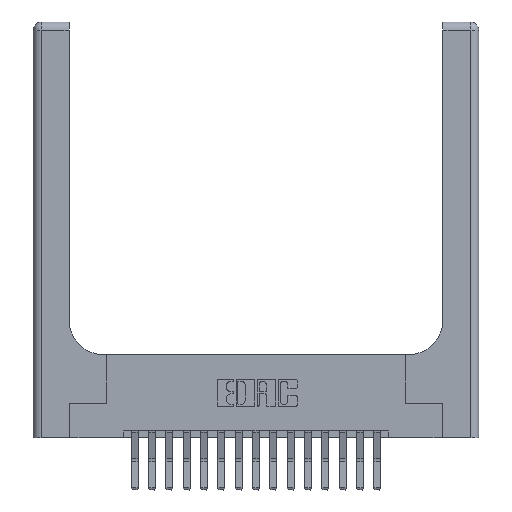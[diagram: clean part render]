
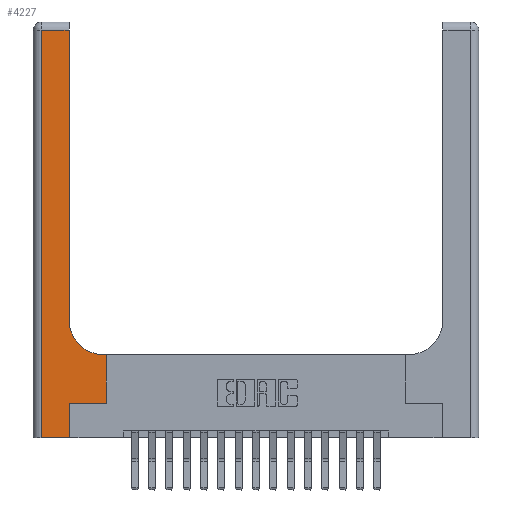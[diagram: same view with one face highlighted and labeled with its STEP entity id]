
A CAD part, top view. The second image highlights one B-rep face of the part: STEP entity #4227.
In plain terms, the highlighted planar face has unit normal (0, 0, 1).
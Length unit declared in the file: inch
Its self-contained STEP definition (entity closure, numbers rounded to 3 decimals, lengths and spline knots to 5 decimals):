
#165 = VERTEX_POINT ( 'NONE', #13885 ) ;
#406 = LINE ( 'NONE', #6337, #1240 ) ;
#1240 = VECTOR ( 'NONE', #18122, 39.37008 ) ;
#1593 = AXIS2_PLACEMENT_3D ( 'NONE', #10858, #15667, #2208 ) ;
#1728 = CARTESIAN_POINT ( 'NONE',  ( 0.265, 0., 0.37 ) ) ;
#1747 = ORIENTED_EDGE ( 'NONE', *, *, #4303, .T. ) ;
#1875 = DIRECTION ( 'NONE',  ( 0., -1., 0. ) ) ;
#2120 = VECTOR ( 'NONE', #1875, 39.37008 ) ;
#2208 = DIRECTION ( 'NONE',  ( 1., 0., 0. ) ) ;
#2814 = ORIENTED_EDGE ( 'NONE', *, *, #10517, .T. ) ;
#3023 = EDGE_CURVE ( 'NONE', #6909, #7137, #11379, .T. ) ;
#3226 = VERTEX_POINT ( 'NONE', #14758 ) ;
#3451 = CARTESIAN_POINT ( 'NONE',  ( 0.528, 0.25, 0.37 ) ) ;
#3509 = DIRECTION ( 'NONE',  ( 1., 0., 0. ) ) ;
#3814 = CARTESIAN_POINT ( 'NONE',  ( 0.26, 0.85, 0.37 ) ) ;
#3913 = DIRECTION ( 'NONE',  ( -1., 0., 0. ) ) ;
#4227 = ADVANCED_FACE ( 'NONE', ( #18217 ), #15396, .F. ) ;
#4303 = EDGE_CURVE ( 'NONE', #10622, #6909, #406, .T. ) ;
#4566 = CARTESIAN_POINT ( 'NONE',  ( 0.06, 2.94, 0.37 ) ) ;
#4660 = ORIENTED_EDGE ( 'NONE', *, *, #9718, .T. ) ;
#5021 = CARTESIAN_POINT ( 'NONE',  ( 0.265, 0.25, 0.37 ) ) ;
#5170 = EDGE_CURVE ( 'NONE', #15595, #15411, #8668, .T. ) ;
#5371 = DIRECTION ( 'NONE',  ( -1., 0., 0. ) ) ;
#5486 = CARTESIAN_POINT ( 'NONE',  ( 0., 2.94, 0.37 ) ) ;
#5850 = EDGE_LOOP ( 'NONE', ( #1747, #8269, #16518, #4660, #14651, #16987, #2814, #18423, #16940 ) ) ;
#6337 = CARTESIAN_POINT ( 'NONE',  ( 0.26, 3., 0.37 ) ) ;
#6622 = CARTESIAN_POINT ( 'NONE',  ( 0.26, 2.94, 0.37 ) ) ;
#6909 = VERTEX_POINT ( 'NONE', #6622 ) ;
#7126 = CARTESIAN_POINT ( 'NONE',  ( 0.26, 0.6, 0.37 ) ) ;
#7137 = VERTEX_POINT ( 'NONE', #4566 ) ;
#7566 = VERTEX_POINT ( 'NONE', #3451 ) ;
#7659 = DIRECTION ( 'NONE',  ( 0., 1., 0. ) ) ;
#7950 = LINE ( 'NONE', #1728, #9952 ) ;
#8118 = CIRCLE ( 'NONE', #1593, 0.25 ) ;
#8269 = ORIENTED_EDGE ( 'NONE', *, *, #3023, .T. ) ;
#8276 = VECTOR ( 'NONE', #11025, 39.37008 ) ;
#8297 = DIRECTION ( 'NONE',  ( 0., 1., 0. ) ) ;
#8310 = CARTESIAN_POINT ( 'NONE',  ( 0.51, 0.6, 0.37 ) ) ;
#8386 = EDGE_CURVE ( 'NONE', #15411, #10622, #8118, .T. ) ;
#8668 = LINE ( 'NONE', #7126, #15766 ) ;
#8744 = EDGE_CURVE ( 'NONE', #165, #11855, #7950, .T. ) ;
#9235 = DIRECTION ( 'NONE',  ( -1., 0., 0. ) ) ;
#9718 = EDGE_CURVE ( 'NONE', #3226, #165, #18427, .T. ) ;
#9952 = VECTOR ( 'NONE', #7659, 39.37008 ) ;
#10517 = EDGE_CURVE ( 'NONE', #7566, #15595, #17178, .T. ) ;
#10622 = VERTEX_POINT ( 'NONE', #3814 ) ;
#10858 = CARTESIAN_POINT ( 'NONE',  ( 0.51, 0.85, 0.37 ) ) ;
#11025 = DIRECTION ( 'NONE',  ( 1., 0., 0. ) ) ;
#11379 = LINE ( 'NONE', #5486, #18909 ) ;
#11855 = VERTEX_POINT ( 'NONE', #12189 ) ;
#12189 = CARTESIAN_POINT ( 'NONE',  ( 0.265, 0.25, 0.37 ) ) ;
#12594 = CARTESIAN_POINT ( 'NONE',  ( 0., 0., 0.37 ) ) ;
#13567 = CARTESIAN_POINT ( 'NONE',  ( 0., 3., 0.37 ) ) ;
#13885 = CARTESIAN_POINT ( 'NONE',  ( 0.265, 0., 0.37 ) ) ;
#13955 = LINE ( 'NONE', #16965, #2120 ) ;
#14616 = VECTOR ( 'NONE', #3509, 39.37008 ) ;
#14651 = ORIENTED_EDGE ( 'NONE', *, *, #8744, .T. ) ;
#14758 = CARTESIAN_POINT ( 'NONE',  ( 0.06, 0., 0.37 ) ) ;
#15134 = AXIS2_PLACEMENT_3D ( 'NONE', #13567, #16574, #9235 ) ;
#15396 = PLANE ( 'NONE',  #15134 ) ;
#15411 = VERTEX_POINT ( 'NONE', #8310 ) ;
#15595 = VERTEX_POINT ( 'NONE', #15928 ) ;
#15667 = DIRECTION ( 'NONE',  ( 0., 0., -1. ) ) ;
#15766 = VECTOR ( 'NONE', #5371, 39.37008 ) ;
#15928 = CARTESIAN_POINT ( 'NONE',  ( 0.528, 0.6, 0.37 ) ) ;
#16498 = VECTOR ( 'NONE', #8297, 39.37008 ) ;
#16518 = ORIENTED_EDGE ( 'NONE', *, *, #18689, .T. ) ;
#16540 = EDGE_CURVE ( 'NONE', #11855, #7566, #18278, .T. ) ;
#16574 = DIRECTION ( 'NONE',  ( 0., 0., -1. ) ) ;
#16940 = ORIENTED_EDGE ( 'NONE', *, *, #8386, .T. ) ;
#16965 = CARTESIAN_POINT ( 'NONE',  ( 0.06, 3., 0.37 ) ) ;
#16987 = ORIENTED_EDGE ( 'NONE', *, *, #16540, .T. ) ;
#17178 = LINE ( 'NONE', #18447, #16498 ) ;
#18122 = DIRECTION ( 'NONE',  ( 0., 1., 0. ) ) ;
#18217 = FACE_OUTER_BOUND ( 'NONE', #5850, .T. ) ;
#18278 = LINE ( 'NONE', #5021, #8276 ) ;
#18423 = ORIENTED_EDGE ( 'NONE', *, *, #5170, .T. ) ;
#18427 = LINE ( 'NONE', #12594, #14616 ) ;
#18447 = CARTESIAN_POINT ( 'NONE',  ( 0.528, 0.25, 0.37 ) ) ;
#18689 = EDGE_CURVE ( 'NONE', #7137, #3226, #13955, .T. ) ;
#18909 = VECTOR ( 'NONE', #3913, 39.37008 ) ;
